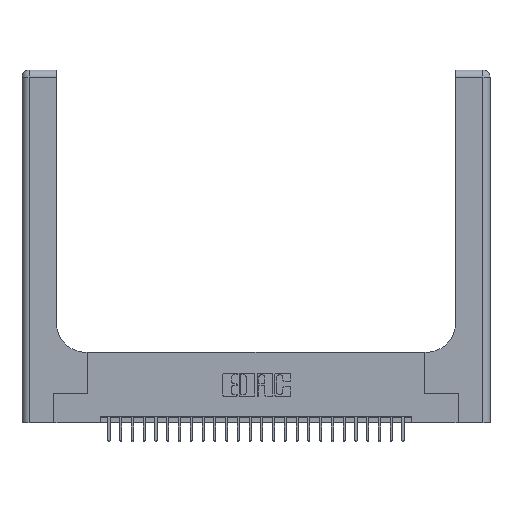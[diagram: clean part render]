
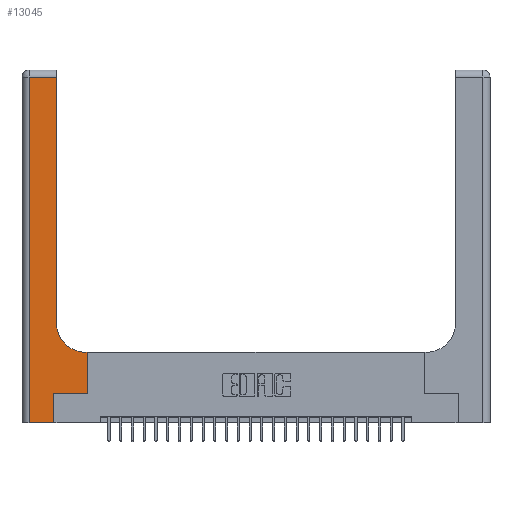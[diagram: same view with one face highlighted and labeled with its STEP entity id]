
A CAD part, top view. The second image highlights one B-rep face of the part: STEP entity #13045.
In plain terms, the highlighted planar face has unit normal (0, 0, 1).
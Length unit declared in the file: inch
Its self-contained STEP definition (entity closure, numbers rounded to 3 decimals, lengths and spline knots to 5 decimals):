
#85 = DIRECTION ( 'NONE',  ( 0., 1., 0. ) ) ;
#107 = CARTESIAN_POINT ( 'NONE',  ( 0.269, 0., 0.37 ) ) ;
#128 = VERTEX_POINT ( 'NONE', #5863 ) ;
#893 = ORIENTED_EDGE ( 'NONE', *, *, #19844, .T. ) ;
#1878 = LINE ( 'NONE', #17291, #19005 ) ;
#2483 = ORIENTED_EDGE ( 'NONE', *, *, #23099, .T. ) ;
#3096 = ORIENTED_EDGE ( 'NONE', *, *, #17021, .T. ) ;
#3141 = LINE ( 'NONE', #10189, #13917 ) ;
#3156 = EDGE_CURVE ( 'NONE', #9963, #21996, #24528, .T. ) ;
#3189 = DIRECTION ( 'NONE',  ( 0., 0., -1. ) ) ;
#3542 = VECTOR ( 'NONE', #8478, 39.37008 ) ;
#4458 = DIRECTION ( 'NONE',  ( 1., 0., 0. ) ) ;
#4561 = DIRECTION ( 'NONE',  ( 0., 0., -1. ) ) ;
#5051 = EDGE_CURVE ( 'NONE', #17640, #26809, #8701, .T. ) ;
#5745 = CARTESIAN_POINT ( 'NONE',  ( 0.06, 3., 0.37 ) ) ;
#5863 = CARTESIAN_POINT ( 'NONE',  ( 0.5585, 0.25, 0.37 ) ) ;
#6078 = CARTESIAN_POINT ( 'NONE',  ( 0.2915, 0.6, 0.37 ) ) ;
#6199 = CARTESIAN_POINT ( 'NONE',  ( 0.5415, 0.6, 0.37 ) ) ;
#7172 = EDGE_CURVE ( 'NONE', #26809, #27531, #16443, .T. ) ;
#7456 = CARTESIAN_POINT ( 'NONE',  ( 0., 3., 0.37 ) ) ;
#7860 = VERTEX_POINT ( 'NONE', #13748 ) ;
#8115 = VECTOR ( 'NONE', #10197, 39.37008 ) ;
#8331 = ORIENTED_EDGE ( 'NONE', *, *, #5051, .T. ) ;
#8418 = VECTOR ( 'NONE', #16484, 39.37008 ) ;
#8478 = DIRECTION ( 'NONE',  ( 1., 0., 0. ) ) ;
#8701 = LINE ( 'NONE', #6078, #19373 ) ;
#8806 = CARTESIAN_POINT ( 'NONE',  ( 0.269, 0., 0.37 ) ) ;
#9487 = VERTEX_POINT ( 'NONE', #107 ) ;
#9587 = LINE ( 'NONE', #23691, #14583 ) ;
#9850 = ORIENTED_EDGE ( 'NONE', *, *, #12221, .T. ) ;
#9963 = VERTEX_POINT ( 'NONE', #21059 ) ;
#10189 = CARTESIAN_POINT ( 'NONE',  ( 0.5585, 0.25, 0.37 ) ) ;
#10197 = DIRECTION ( 'NONE',  ( 0., -1., 0. ) ) ;
#10618 = CARTESIAN_POINT ( 'NONE',  ( 0.269, 0.25, 0.37 ) ) ;
#11090 = EDGE_LOOP ( 'NONE', ( #19037, #893, #15181, #9850, #3096, #17549, #2483, #8331, #24406 ) ) ;
#12221 = EDGE_CURVE ( 'NONE', #21996, #9487, #1878, .T. ) ;
#12775 = CARTESIAN_POINT ( 'NONE',  ( 0.269, 0.25, 0.37 ) ) ;
#13045 = ADVANCED_FACE ( 'NONE', ( #16322 ), #15961, .F. ) ;
#13052 = CARTESIAN_POINT ( 'NONE',  ( 0.06, 0., 0.37 ) ) ;
#13103 = VECTOR ( 'NONE', #25929, 39.37008 ) ;
#13748 = CARTESIAN_POINT ( 'NONE',  ( 0.2915, 2.94, 0.37 ) ) ;
#13917 = VECTOR ( 'NONE', #27293, 39.37008 ) ;
#14154 = EDGE_CURVE ( 'NONE', #27531, #7860, #9587, .T. ) ;
#14583 = VECTOR ( 'NONE', #85, 39.37008 ) ;
#15181 = ORIENTED_EDGE ( 'NONE', *, *, #3156, .T. ) ;
#15961 = PLANE ( 'NONE',  #20504 ) ;
#16322 = FACE_OUTER_BOUND ( 'NONE', #11090, .T. ) ;
#16443 = CIRCLE ( 'NONE', #23462, 0.25 ) ;
#16484 = DIRECTION ( 'NONE',  ( -1., 0., 0. ) ) ;
#17021 = EDGE_CURVE ( 'NONE', #9487, #23851, #23152, .T. ) ;
#17149 = CARTESIAN_POINT ( 'NONE',  ( 0.5585, 0.6, 0.37 ) ) ;
#17291 = CARTESIAN_POINT ( 'NONE',  ( 0., 0., 0.37 ) ) ;
#17395 = CARTESIAN_POINT ( 'NONE',  ( 0.5415, 0.85, 0.37 ) ) ;
#17549 = ORIENTED_EDGE ( 'NONE', *, *, #21913, .T. ) ;
#17640 = VERTEX_POINT ( 'NONE', #17149 ) ;
#18136 = CARTESIAN_POINT ( 'NONE',  ( 0.2915, 0.85, 0.37 ) ) ;
#18203 = DIRECTION ( 'NONE',  ( -1., 0., 0. ) ) ;
#18999 = DIRECTION ( 'NONE',  ( -1., 0., 0. ) ) ;
#19005 = VECTOR ( 'NONE', #4458, 39.37008 ) ;
#19037 = ORIENTED_EDGE ( 'NONE', *, *, #14154, .T. ) ;
#19373 = VECTOR ( 'NONE', #18999, 39.37008 ) ;
#19552 = DIRECTION ( 'NONE',  ( 1., 0., 0. ) ) ;
#19844 = EDGE_CURVE ( 'NONE', #7860, #9963, #20454, .T. ) ;
#20454 = LINE ( 'NONE', #25035, #8418 ) ;
#20504 = AXIS2_PLACEMENT_3D ( 'NONE', #7456, #3189, #18203 ) ;
#20669 = LINE ( 'NONE', #12775, #3542 ) ;
#21059 = CARTESIAN_POINT ( 'NONE',  ( 0.06, 2.94, 0.37 ) ) ;
#21913 = EDGE_CURVE ( 'NONE', #23851, #128, #20669, .T. ) ;
#21996 = VERTEX_POINT ( 'NONE', #13052 ) ;
#23099 = EDGE_CURVE ( 'NONE', #128, #17640, #3141, .T. ) ;
#23152 = LINE ( 'NONE', #8806, #13103 ) ;
#23462 = AXIS2_PLACEMENT_3D ( 'NONE', #17395, #4561, #19552 ) ;
#23691 = CARTESIAN_POINT ( 'NONE',  ( 0.2915, 3., 0.37 ) ) ;
#23851 = VERTEX_POINT ( 'NONE', #10618 ) ;
#24406 = ORIENTED_EDGE ( 'NONE', *, *, #7172, .T. ) ;
#24528 = LINE ( 'NONE', #5745, #8115 ) ;
#25035 = CARTESIAN_POINT ( 'NONE',  ( 0., 2.94, 0.37 ) ) ;
#25929 = DIRECTION ( 'NONE',  ( 0., 1., 0. ) ) ;
#26809 = VERTEX_POINT ( 'NONE', #6199 ) ;
#27293 = DIRECTION ( 'NONE',  ( 0., 1., 0. ) ) ;
#27531 = VERTEX_POINT ( 'NONE', #18136 ) ;
